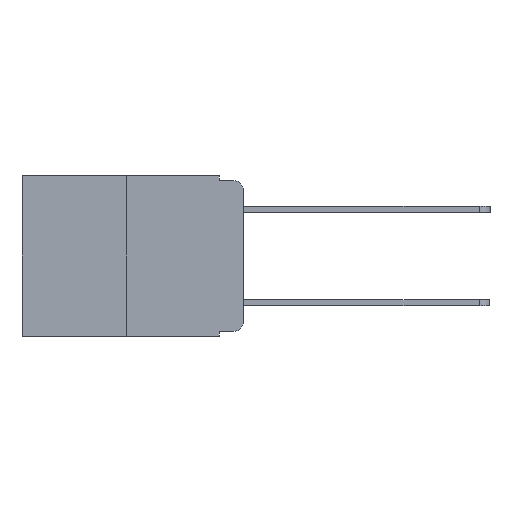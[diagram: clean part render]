
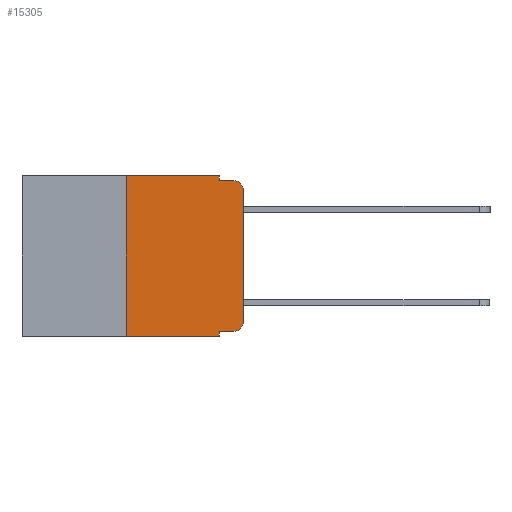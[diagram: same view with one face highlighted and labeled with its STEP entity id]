
A CAD part, left-side view. The second image highlights one B-rep face of the part: STEP entity #15305.
In plain terms, the highlighted planar face has unit normal (-1, 0, 0).
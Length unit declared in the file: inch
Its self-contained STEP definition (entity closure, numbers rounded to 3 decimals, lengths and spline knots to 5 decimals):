
#136 = EDGE_CURVE ( 'NONE', #20705, #13155, #10744, .T. ) ;
#327 = DIRECTION ( 'NONE',  ( 0., -1., 0. ) ) ;
#375 = VERTEX_POINT ( 'NONE', #12220 ) ;
#499 = VERTEX_POINT ( 'NONE', #10319 ) ;
#508 = EDGE_CURVE ( 'NONE', #25085, #19137, #17449, .T. ) ;
#579 = CARTESIAN_POINT ( 'NONE',  ( 0., 0.051, -0.343 ) ) ;
#582 = CIRCLE ( 'NONE', #15680, 0.02 ) ;
#814 = DIRECTION ( 'NONE',  ( -1., 0., 0. ) ) ;
#882 = VECTOR ( 'NONE', #25397, 39.37008 ) ;
#1175 = VECTOR ( 'NONE', #10911, 39.37008 ) ;
#1249 = VECTOR ( 'NONE', #4923, 39.37008 ) ;
#1660 = CARTESIAN_POINT ( 'NONE',  ( 0., 0.051, 0. ) ) ;
#1750 = DIRECTION ( 'NONE',  ( 1., 0., 0. ) ) ;
#1821 = EDGE_LOOP ( 'NONE', ( #11364, #6228, #24657, #6595, #11773, #5551, #14794, #16294, #4134, #21350 ) ) ;
#2917 = CARTESIAN_POINT ( 'NONE',  ( 0., 0.02, -0.01 ) ) ;
#2940 = CARTESIAN_POINT ( 'NONE',  ( 0., 0.02, -0.333 ) ) ;
#3460 = EDGE_CURVE ( 'NONE', #499, #16745, #582, .T. ) ;
#3959 = CARTESIAN_POINT ( 'NONE',  ( 0., 0.051, -0.333 ) ) ;
#4134 = ORIENTED_EDGE ( 'NONE', *, *, #508, .T. ) ;
#4923 = DIRECTION ( 'NONE',  ( 0., -1., 0. ) ) ;
#5046 = CARTESIAN_POINT ( 'NONE',  ( 0., 0.02, -0.03 ) ) ;
#5551 = ORIENTED_EDGE ( 'NONE', *, *, #136, .F. ) ;
#5561 = CARTESIAN_POINT ( 'NONE',  ( 0., 0.25, 0. ) ) ;
#5685 = AXIS2_PLACEMENT_3D ( 'NONE', #13122, #814, #15182 ) ;
#5791 = VERTEX_POINT ( 'NONE', #1660 ) ;
#6013 = LINE ( 'NONE', #18607, #6640 ) ;
#6228 = ORIENTED_EDGE ( 'NONE', *, *, #3460, .T. ) ;
#6595 = ORIENTED_EDGE ( 'NONE', *, *, #18573, .F. ) ;
#6640 = VECTOR ( 'NONE', #10219, 39.37008 ) ;
#7073 = DIRECTION ( 'NONE',  ( 0., 0., -1. ) ) ;
#7380 = LINE ( 'NONE', #7818, #17654 ) ;
#7521 = AXIS2_PLACEMENT_3D ( 'NONE', #24266, #1750, #16085 ) ;
#7818 = CARTESIAN_POINT ( 'NONE',  ( 0., 0.473, -0.343 ) ) ;
#8355 = DIRECTION ( 'NONE',  ( 0., 0., 1. ) ) ;
#8937 = EDGE_CURVE ( 'NONE', #9517, #499, #15157, .T. ) ;
#9517 = VERTEX_POINT ( 'NONE', #24170 ) ;
#9926 = CARTESIAN_POINT ( 'NONE',  ( 0., 0., 0. ) ) ;
#10072 = EDGE_CURVE ( 'NONE', #20705, #17838, #7380, .T. ) ;
#10219 = DIRECTION ( 'NONE',  ( 0., -1., 0. ) ) ;
#10319 = CARTESIAN_POINT ( 'NONE',  ( 0., 0., -0.03 ) ) ;
#10744 = LINE ( 'NONE', #5561, #14919 ) ;
#10911 = DIRECTION ( 'NONE',  ( 0., 0., -1. ) ) ;
#11364 = ORIENTED_EDGE ( 'NONE', *, *, #8937, .T. ) ;
#11746 = CIRCLE ( 'NONE', #5685, 0.02 ) ;
#11773 = ORIENTED_EDGE ( 'NONE', *, *, #17907, .F. ) ;
#11832 = LINE ( 'NONE', #21387, #882 ) ;
#12008 = VECTOR ( 'NONE', #327, 39.37008 ) ;
#12220 = CARTESIAN_POINT ( 'NONE',  ( 0., 0.051, -0.01 ) ) ;
#12568 = EDGE_CURVE ( 'NONE', #25085, #17838, #23032, .T. ) ;
#13072 = EDGE_CURVE ( 'NONE', #375, #16745, #6013, .T. ) ;
#13122 = CARTESIAN_POINT ( 'NONE',  ( 0., 0.02, -0.313 ) ) ;
#13155 = VERTEX_POINT ( 'NONE', #16672 ) ;
#13480 = LINE ( 'NONE', #17185, #1249 ) ;
#13879 = VECTOR ( 'NONE', #26335, 39.37008 ) ;
#14586 = FACE_OUTER_BOUND ( 'NONE', #1821, .T. ) ;
#14794 = ORIENTED_EDGE ( 'NONE', *, *, #10072, .T. ) ;
#14919 = VECTOR ( 'NONE', #8355, 39.37008 ) ;
#15038 = CARTESIAN_POINT ( 'NONE',  ( 0., 0.051, 0. ) ) ;
#15157 = LINE ( 'NONE', #9926, #13879 ) ;
#15182 = DIRECTION ( 'NONE',  ( 0., 0., -1. ) ) ;
#15305 = ADVANCED_FACE ( 'NONE', ( #14586 ), #26308, .F. ) ;
#15680 = AXIS2_PLACEMENT_3D ( 'NONE', #5046, #19375, #7073 ) ;
#16085 = DIRECTION ( 'NONE',  ( 0., 0., -1. ) ) ;
#16294 = ORIENTED_EDGE ( 'NONE', *, *, #12568, .F. ) ;
#16660 = CARTESIAN_POINT ( 'NONE',  ( 0., 0.051, -0.333 ) ) ;
#16672 = CARTESIAN_POINT ( 'NONE',  ( 0., 0.25, 0. ) ) ;
#16745 = VERTEX_POINT ( 'NONE', #2917 ) ;
#17185 = CARTESIAN_POINT ( 'NONE',  ( 0., 0.473, 0. ) ) ;
#17449 = LINE ( 'NONE', #3959, #12008 ) ;
#17654 = VECTOR ( 'NONE', #20128, 39.37008 ) ;
#17838 = VERTEX_POINT ( 'NONE', #579 ) ;
#17907 = EDGE_CURVE ( 'NONE', #13155, #5791, #13480, .T. ) ;
#18573 = EDGE_CURVE ( 'NONE', #5791, #375, #11832, .T. ) ;
#18607 = CARTESIAN_POINT ( 'NONE',  ( 0., 0.051, -0.01 ) ) ;
#19137 = VERTEX_POINT ( 'NONE', #2940 ) ;
#19375 = DIRECTION ( 'NONE',  ( -1., 0., 0. ) ) ;
#20128 = DIRECTION ( 'NONE',  ( 0., -1., 0. ) ) ;
#20182 = CARTESIAN_POINT ( 'NONE',  ( 0., 0.25, -0.343 ) ) ;
#20705 = VERTEX_POINT ( 'NONE', #20182 ) ;
#21350 = ORIENTED_EDGE ( 'NONE', *, *, #25764, .T. ) ;
#21387 = CARTESIAN_POINT ( 'NONE',  ( 0., 0.051, 0. ) ) ;
#23032 = LINE ( 'NONE', #15038, #1175 ) ;
#24170 = CARTESIAN_POINT ( 'NONE',  ( 0., 0., -0.313 ) ) ;
#24266 = CARTESIAN_POINT ( 'NONE',  ( 0., 0.473, 0. ) ) ;
#24657 = ORIENTED_EDGE ( 'NONE', *, *, #13072, .F. ) ;
#25085 = VERTEX_POINT ( 'NONE', #16660 ) ;
#25397 = DIRECTION ( 'NONE',  ( 0., 0., -1. ) ) ;
#25764 = EDGE_CURVE ( 'NONE', #19137, #9517, #11746, .T. ) ;
#26308 = PLANE ( 'NONE',  #7521 ) ;
#26335 = DIRECTION ( 'NONE',  ( 0., 0., 1. ) ) ;
